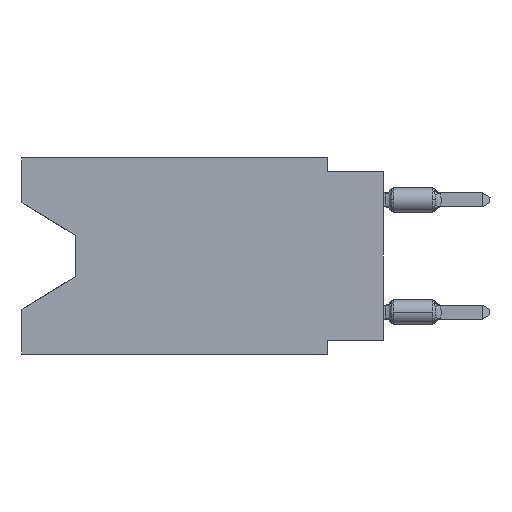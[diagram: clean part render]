
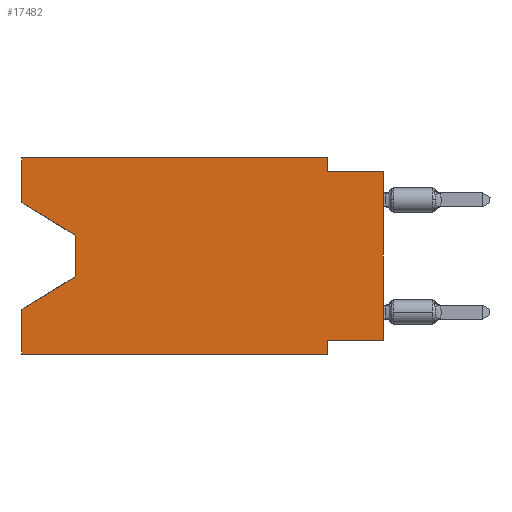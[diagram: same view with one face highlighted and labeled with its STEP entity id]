
A CAD part, left-side view. The second image highlights one B-rep face of the part: STEP entity #17482.
In plain terms, the highlighted planar face has unit normal (-1, 0, 0).
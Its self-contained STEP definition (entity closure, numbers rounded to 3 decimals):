
#147 = VERTEX_POINT ( 'NONE', #1891 ) ;
#190 = CARTESIAN_POINT ( 'NONE',  ( 0., 2.54, 0. ) ) ;
#1018 = DIRECTION ( 'NONE',  ( 0., 0., -1. ) ) ;
#1023 = EDGE_CURVE ( 'NONE', #42263, #43337, #27589, .T. ) ;
#1266 = VERTEX_POINT ( 'NONE', #32097 ) ;
#1891 = CARTESIAN_POINT ( 'NONE',  ( 0., 16.383, -6.852 ) ) ;
#2070 = ORIENTED_EDGE ( 'NONE', *, *, #1023, .F. ) ;
#2244 = DIRECTION ( 'NONE',  ( 0., 0.855, -0.519 ) ) ;
#3077 = CARTESIAN_POINT ( 'NONE',  ( 0., 16.383, -8.89 ) ) ;
#3696 = DIRECTION ( 'NONE',  ( 0., -1., 0. ) ) ;
#4731 = CARTESIAN_POINT ( 'NONE',  ( 0., 0., -0.635 ) ) ;
#4919 = EDGE_CURVE ( 'NONE', #21902, #42263, #50046, .T. ) ;
#5338 = DIRECTION ( 'NONE',  ( 0., 0., 1. ) ) ;
#6816 = VERTEX_POINT ( 'NONE', #8792 ) ;
#7506 = DIRECTION ( 'NONE',  ( 0., 1., 0. ) ) ;
#7523 = CARTESIAN_POINT ( 'NONE',  ( 0., 16.383, 0. ) ) ;
#8053 = DIRECTION ( 'NONE',  ( 0., -1., 0. ) ) ;
#8792 = CARTESIAN_POINT ( 'NONE',  ( 0., 2.54, -8.89 ) ) ;
#9191 = CARTESIAN_POINT ( 'NONE',  ( 0., 13.97, -3.505 ) ) ;
#9273 = VERTEX_POINT ( 'NONE', #32849 ) ;
#9291 = ORIENTED_EDGE ( 'NONE', *, *, #12213, .F. ) ;
#9575 = CARTESIAN_POINT ( 'NONE',  ( 0., 2.54, -8.255 ) ) ;
#11157 = LINE ( 'NONE', #42398, #18153 ) ;
#11541 = VERTEX_POINT ( 'NONE', #37600 ) ;
#12213 = EDGE_CURVE ( 'NONE', #43337, #34552, #11157, .T. ) ;
#13752 = CARTESIAN_POINT ( 'NONE',  ( 0., 13.97, -5.385 ) ) ;
#14049 = DIRECTION ( 'NONE',  ( 0., -0.855, -0.519 ) ) ;
#14725 = EDGE_CURVE ( 'NONE', #11541, #1266, #36625, .T. ) ;
#14938 = ORIENTED_EDGE ( 'NONE', *, *, #4919, .F. ) ;
#15643 = EDGE_CURVE ( 'NONE', #49955, #147, #36499, .T. ) ;
#16130 = CARTESIAN_POINT ( 'NONE',  ( 0., 0., 0. ) ) ;
#16341 = EDGE_CURVE ( 'NONE', #1266, #147, #21683, .T. ) ;
#16863 = VECTOR ( 'NONE', #8053, 1000. ) ;
#17022 = CARTESIAN_POINT ( 'NONE',  ( 0., 16.383, 0. ) ) ;
#17314 = VERTEX_POINT ( 'NONE', #20984 ) ;
#17436 = EDGE_CURVE ( 'NONE', #17314, #11541, #22236, .T. ) ;
#17482 = ADVANCED_FACE ( 'NONE', ( #26101 ), #41219, .F. ) ;
#17961 = EDGE_CURVE ( 'NONE', #9273, #34725, #34410, .T. ) ;
#18126 = VECTOR ( 'NONE', #5338, 1000. ) ;
#18153 = VECTOR ( 'NONE', #22904, 1000. ) ;
#18400 = DIRECTION ( 'NONE',  ( 1., 0., 0. ) ) ;
#20306 = VECTOR ( 'NONE', #3696, 1000. ) ;
#20388 = ORIENTED_EDGE ( 'NONE', *, *, #15643, .F. ) ;
#20609 = CARTESIAN_POINT ( 'NONE',  ( 0., 16.383, 0. ) ) ;
#20984 = CARTESIAN_POINT ( 'NONE',  ( 0., 16.383, -2.038 ) ) ;
#21683 = LINE ( 'NONE', #13752, #35294 ) ;
#21749 = DIRECTION ( 'NONE',  ( 0., 0., -1. ) ) ;
#21902 = VERTEX_POINT ( 'NONE', #20609 ) ;
#21927 = DIRECTION ( 'NONE',  ( 0., 0., -1. ) ) ;
#22128 = CARTESIAN_POINT ( 'NONE',  ( 0., 16.383, 0. ) ) ;
#22236 = LINE ( 'NONE', #29945, #26363 ) ;
#22904 = DIRECTION ( 'NONE',  ( 0., -1., 0. ) ) ;
#23039 = ORIENTED_EDGE ( 'NONE', *, *, #14725, .T. ) ;
#23413 = LINE ( 'NONE', #24176, #16863 ) ;
#23484 = ORIENTED_EDGE ( 'NONE', *, *, #17961, .F. ) ;
#23503 = EDGE_CURVE ( 'NONE', #49955, #6816, #23413, .T. ) ;
#23974 = DIRECTION ( 'NONE',  ( 0., 0., -1. ) ) ;
#24142 = ORIENTED_EDGE ( 'NONE', *, *, #49044, .F. ) ;
#24176 = CARTESIAN_POINT ( 'NONE',  ( 0., 16.383, -8.89 ) ) ;
#25084 = VECTOR ( 'NONE', #32646, 1000. ) ;
#25741 = DIRECTION ( 'NONE',  ( 0., 0., 1. ) ) ;
#26101 = FACE_OUTER_BOUND ( 'NONE', #29287, .T. ) ;
#26363 = VECTOR ( 'NONE', #14049, 1000. ) ;
#27589 = LINE ( 'NONE', #47294, #32739 ) ;
#28878 = VECTOR ( 'NONE', #25741, 1000. ) ;
#29287 = EDGE_LOOP ( 'NONE', ( #39629, #23039, #50110, #20388, #41438, #37599, #23484, #40286, #9291, #2070, #14938, #24142 ) ) ;
#29868 = CARTESIAN_POINT ( 'NONE',  ( 0., 2.54, -8.89 ) ) ;
#29931 = CARTESIAN_POINT ( 'NONE',  ( 0., 2.54, -0.635 ) ) ;
#29945 = CARTESIAN_POINT ( 'NONE',  ( 0., 16.383, -2.038 ) ) ;
#32097 = CARTESIAN_POINT ( 'NONE',  ( 0., 13.97, -5.385 ) ) ;
#32646 = DIRECTION ( 'NONE',  ( 0., 0., 1. ) ) ;
#32739 = VECTOR ( 'NONE', #23974, 1000. ) ;
#32849 = CARTESIAN_POINT ( 'NONE',  ( 0., 0., -8.255 ) ) ;
#33961 = LINE ( 'NONE', #29868, #35531 ) ;
#34410 = LINE ( 'NONE', #42590, #40217 ) ;
#34552 = VERTEX_POINT ( 'NONE', #4731 ) ;
#34725 = VERTEX_POINT ( 'NONE', #9575 ) ;
#35294 = VECTOR ( 'NONE', #2244, 1000. ) ;
#35531 = VECTOR ( 'NONE', #21927, 1000. ) ;
#36499 = LINE ( 'NONE', #17022, #25084 ) ;
#36625 = LINE ( 'NONE', #9191, #47097 ) ;
#37599 = ORIENTED_EDGE ( 'NONE', *, *, #43740, .F. ) ;
#37600 = CARTESIAN_POINT ( 'NONE',  ( 0., 13.97, -3.505 ) ) ;
#37624 = CARTESIAN_POINT ( 'NONE',  ( 0., 16.383, 0. ) ) ;
#39629 = ORIENTED_EDGE ( 'NONE', *, *, #17436, .T. ) ;
#40217 = VECTOR ( 'NONE', #7506, 1000. ) ;
#40286 = ORIENTED_EDGE ( 'NONE', *, *, #40744, .T. ) ;
#40744 = EDGE_CURVE ( 'NONE', #9273, #34552, #48344, .T. ) ;
#41219 = PLANE ( 'NONE',  #49161 ) ;
#41438 = ORIENTED_EDGE ( 'NONE', *, *, #23503, .T. ) ;
#42263 = VERTEX_POINT ( 'NONE', #190 ) ;
#42398 = CARTESIAN_POINT ( 'NONE',  ( 0., 0., -0.635 ) ) ;
#42590 = CARTESIAN_POINT ( 'NONE',  ( 0., 0., -8.255 ) ) ;
#43337 = VERTEX_POINT ( 'NONE', #29931 ) ;
#43740 = EDGE_CURVE ( 'NONE', #34725, #6816, #33961, .T. ) ;
#45694 = LINE ( 'NONE', #22128, #28878 ) ;
#47097 = VECTOR ( 'NONE', #1018, 1000. ) ;
#47294 = CARTESIAN_POINT ( 'NONE',  ( 0., 2.54, 0. ) ) ;
#48344 = LINE ( 'NONE', #16130, #18126 ) ;
#49044 = EDGE_CURVE ( 'NONE', #17314, #21902, #45694, .T. ) ;
#49161 = AXIS2_PLACEMENT_3D ( 'NONE', #37624, #18400, #21749 ) ;
#49955 = VERTEX_POINT ( 'NONE', #3077 ) ;
#50046 = LINE ( 'NONE', #7523, #20306 ) ;
#50110 = ORIENTED_EDGE ( 'NONE', *, *, #16341, .T. ) ;
